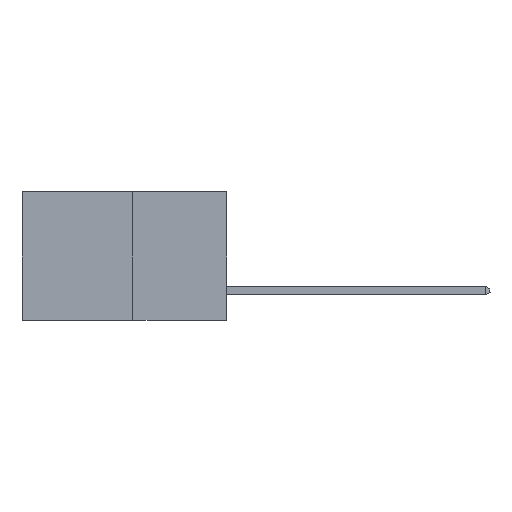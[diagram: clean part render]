
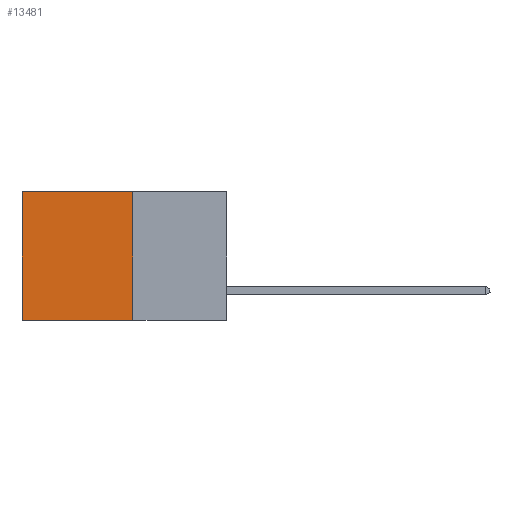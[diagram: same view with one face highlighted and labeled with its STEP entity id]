
A CAD part, left-side view. The second image highlights one B-rep face of the part: STEP entity #13481.
In plain terms, the highlighted planar face has unit normal (-1, 0, 0).
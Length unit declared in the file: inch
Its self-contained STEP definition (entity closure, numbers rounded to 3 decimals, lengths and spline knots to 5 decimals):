
#1186 = EDGE_CURVE ( 'NONE', #25749, #9031, #23673, .T. ) ;
#1414 = DIRECTION ( 'NONE',  ( 0., 0., -1. ) ) ;
#3166 = PLANE ( 'NONE',  #19276 ) ;
#4322 = VECTOR ( 'NONE', #1414, 39.37008 ) ;
#4342 = VECTOR ( 'NONE', #23145, 39.37008 ) ;
#4573 = DIRECTION ( 'NONE',  ( 0., 1., 0. ) ) ;
#5730 = CARTESIAN_POINT ( 'NONE',  ( 0.277, 0.59, -0.37 ) ) ;
#5934 = FACE_OUTER_BOUND ( 'NONE', #13864, .T. ) ;
#6386 = CARTESIAN_POINT ( 'NONE',  ( 0.277, 0.27, -0.37 ) ) ;
#6502 = VECTOR ( 'NONE', #4573, 39.37008 ) ;
#8593 = ORIENTED_EDGE ( 'NONE', *, *, #14166, .F. ) ;
#9031 = VERTEX_POINT ( 'NONE', #9351 ) ;
#9351 = CARTESIAN_POINT ( 'NONE',  ( 0.277, 0.59, -0.37 ) ) ;
#10051 = CARTESIAN_POINT ( 'NONE',  ( 0.277, 0.27, -0.37 ) ) ;
#10363 = CARTESIAN_POINT ( 'NONE',  ( 0.277, 0.27, 0. ) ) ;
#10590 = VECTOR ( 'NONE', #21431, 39.37008 ) ;
#10754 = LINE ( 'NONE', #12213, #4342 ) ;
#11596 = EDGE_CURVE ( 'NONE', #26634, #9031, #22233, .T. ) ;
#12213 = CARTESIAN_POINT ( 'NONE',  ( 0.277, 0.27, 0. ) ) ;
#12226 = DIRECTION ( 'NONE',  ( 0., 0., -1. ) ) ;
#13481 = ADVANCED_FACE ( 'NONE', ( #5934 ), #3166, .F. ) ;
#13864 = EDGE_LOOP ( 'NONE', ( #16059, #22421, #8593, #27773 ) ) ;
#14166 = EDGE_CURVE ( 'NONE', #26563, #25749, #27079, .T. ) ;
#16059 = ORIENTED_EDGE ( 'NONE', *, *, #11596, .T. ) ;
#19276 = AXIS2_PLACEMENT_3D ( 'NONE', #10051, #25124, #12226 ) ;
#19283 = CARTESIAN_POINT ( 'NONE',  ( 0.277, 0.27, -0.37 ) ) ;
#19337 = CARTESIAN_POINT ( 'NONE',  ( 0.277, 0.59, 0. ) ) ;
#21431 = DIRECTION ( 'NONE',  ( 0., 0., -1. ) ) ;
#21998 = CARTESIAN_POINT ( 'NONE',  ( 0.277, 0.27, -0.37 ) ) ;
#22233 = LINE ( 'NONE', #5730, #4322 ) ;
#22421 = ORIENTED_EDGE ( 'NONE', *, *, #1186, .F. ) ;
#23067 = EDGE_CURVE ( 'NONE', #26563, #26634, #10754, .T. ) ;
#23145 = DIRECTION ( 'NONE',  ( 0., 1., 0. ) ) ;
#23673 = LINE ( 'NONE', #21998, #6502 ) ;
#25124 = DIRECTION ( 'NONE',  ( 1., 0., 0. ) ) ;
#25749 = VERTEX_POINT ( 'NONE', #19283 ) ;
#26563 = VERTEX_POINT ( 'NONE', #10363 ) ;
#26634 = VERTEX_POINT ( 'NONE', #19337 ) ;
#27079 = LINE ( 'NONE', #6386, #10590 ) ;
#27773 = ORIENTED_EDGE ( 'NONE', *, *, #23067, .T. ) ;
